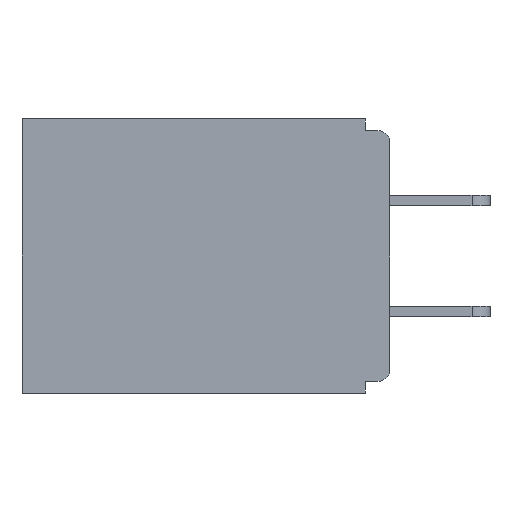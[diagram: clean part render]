
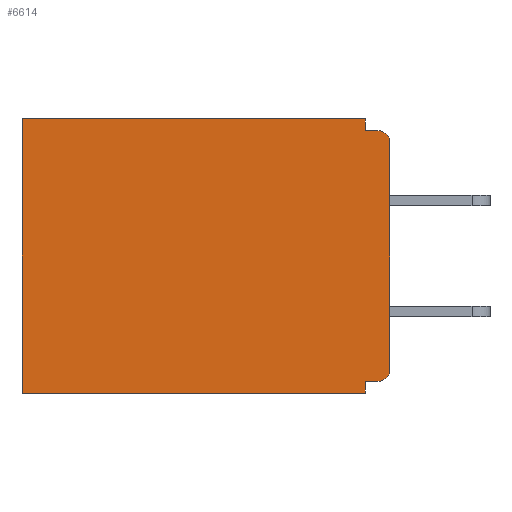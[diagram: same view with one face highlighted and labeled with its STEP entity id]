
A CAD part, left-side view. The second image highlights one B-rep face of the part: STEP entity #6614.
In plain terms, the highlighted planar face has unit normal (-1, 0, 0).
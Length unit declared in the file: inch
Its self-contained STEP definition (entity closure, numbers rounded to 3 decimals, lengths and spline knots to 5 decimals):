
#872 = AXIS2_PLACEMENT_3D ( 'NONE', #21377, #1498, #17815 ) ;
#1228 = DIRECTION ( 'NONE',  ( 0., 1., 0. ) ) ;
#1498 = DIRECTION ( 'NONE',  ( -1., 0., 0. ) ) ;
#2060 = EDGE_LOOP ( 'NONE', ( #9088, #4891, #14933, #8256, #21870, #21727, #25203, #8234, #14014, #2241 ) ) ;
#2160 = VERTEX_POINT ( 'NONE', #13842 ) ;
#2241 = ORIENTED_EDGE ( 'NONE', *, *, #13747, .F. ) ;
#2498 = DIRECTION ( 'NONE',  ( 0., 0., -1. ) ) ;
#3369 = VECTOR ( 'NONE', #23822, 39.37008 ) ;
#3476 = DIRECTION ( 'NONE',  ( 1., 0., 0. ) ) ;
#3759 = VERTEX_POINT ( 'NONE', #11591 ) ;
#3927 = CARTESIAN_POINT ( 'NONE',  ( 0.298, 0., -0.328 ) ) ;
#4252 = EDGE_CURVE ( 'NONE', #3759, #8314, #20548, .T. ) ;
#4494 = LINE ( 'NONE', #11428, #9475 ) ;
#4512 = CARTESIAN_POINT ( 'NONE',  ( 0.298, 0.015, -0.03 ) ) ;
#4557 = EDGE_CURVE ( 'NONE', #3759, #5519, #8683, .T. ) ;
#4628 = LINE ( 'NONE', #11725, #3369 ) ;
#4753 = CARTESIAN_POINT ( 'NONE',  ( 0.298, 0.46, 0. ) ) ;
#4891 = ORIENTED_EDGE ( 'NONE', *, *, #8726, .F. ) ;
#5317 = PLANE ( 'NONE',  #8557 ) ;
#5519 = VERTEX_POINT ( 'NONE', #7289 ) ;
#6614 = ADVANCED_FACE ( 'NONE', ( #15911 ), #5317, .F. ) ;
#7010 = EDGE_CURVE ( 'NONE', #22386, #8711, #13099, .T. ) ;
#7146 = AXIS2_PLACEMENT_3D ( 'NONE', #4512, #18550, #20522 ) ;
#7289 = CARTESIAN_POINT ( 'NONE',  ( 0.298, 0.031, -0.328 ) ) ;
#7302 = DIRECTION ( 'NONE',  ( 0., 0., -1. ) ) ;
#7471 = DIRECTION ( 'NONE',  ( 0., 0., -1. ) ) ;
#7636 = VECTOR ( 'NONE', #1228, 39.37008 ) ;
#8234 = ORIENTED_EDGE ( 'NONE', *, *, #4557, .F. ) ;
#8256 = ORIENTED_EDGE ( 'NONE', *, *, #20867, .T. ) ;
#8286 = LINE ( 'NONE', #14314, #24186 ) ;
#8314 = VERTEX_POINT ( 'NONE', #20433 ) ;
#8557 = AXIS2_PLACEMENT_3D ( 'NONE', #13546, #3476, #7471 ) ;
#8588 = LINE ( 'NONE', #25038, #7636 ) ;
#8683 = LINE ( 'NONE', #3927, #24899 ) ;
#8711 = VERTEX_POINT ( 'NONE', #19725 ) ;
#8726 = EDGE_CURVE ( 'NONE', #21543, #16826, #4628, .T. ) ;
#9088 = ORIENTED_EDGE ( 'NONE', *, *, #20347, .T. ) ;
#9347 = VERTEX_POINT ( 'NONE', #11009 ) ;
#9475 = VECTOR ( 'NONE', #17098, 39.37008 ) ;
#10661 = CARTESIAN_POINT ( 'NONE',  ( 0.298, 0.031, -0.343 ) ) ;
#11009 = CARTESIAN_POINT ( 'NONE',  ( 0.298, 0.46, 0. ) ) ;
#11428 = CARTESIAN_POINT ( 'NONE',  ( 0.298, 0., 0. ) ) ;
#11591 = CARTESIAN_POINT ( 'NONE',  ( 0.298, 0.015, -0.328 ) ) ;
#11686 = EDGE_CURVE ( 'NONE', #9347, #8711, #22696, .T. ) ;
#11725 = CARTESIAN_POINT ( 'NONE',  ( 0.298, 0., -0.015 ) ) ;
#12074 = CARTESIAN_POINT ( 'NONE',  ( 0.298, 0., -0.343 ) ) ;
#13099 = LINE ( 'NONE', #12074, #18102 ) ;
#13546 = CARTESIAN_POINT ( 'NONE',  ( 0.298, 0., 0. ) ) ;
#13747 = EDGE_CURVE ( 'NONE', #2160, #8314, #4494, .T. ) ;
#13807 = DIRECTION ( 'NONE',  ( 0., 1., 0. ) ) ;
#13842 = CARTESIAN_POINT ( 'NONE',  ( 0.298, 0., -0.03 ) ) ;
#14014 = ORIENTED_EDGE ( 'NONE', *, *, #4252, .T. ) ;
#14314 = CARTESIAN_POINT ( 'NONE',  ( 0.298, 0.031, -0.343 ) ) ;
#14933 = ORIENTED_EDGE ( 'NONE', *, *, #20462, .F. ) ;
#15702 = VERTEX_POINT ( 'NONE', #16570 ) ;
#15754 = CIRCLE ( 'NONE', #7146, 0.015 ) ;
#15903 = VECTOR ( 'NONE', #7302, 39.37008 ) ;
#15911 = FACE_OUTER_BOUND ( 'NONE', #2060, .T. ) ;
#16570 = CARTESIAN_POINT ( 'NONE',  ( 0.298, 0.031, 0. ) ) ;
#16826 = VERTEX_POINT ( 'NONE', #17215 ) ;
#17098 = DIRECTION ( 'NONE',  ( 0., 0., -1. ) ) ;
#17215 = CARTESIAN_POINT ( 'NONE',  ( 0.298, 0.015, -0.015 ) ) ;
#17415 = VECTOR ( 'NONE', #24261, 39.37008 ) ;
#17815 = DIRECTION ( 'NONE',  ( 0., 0., -1. ) ) ;
#18102 = VECTOR ( 'NONE', #13807, 39.37008 ) ;
#18550 = DIRECTION ( 'NONE',  ( -1., 0., 0. ) ) ;
#19725 = CARTESIAN_POINT ( 'NONE',  ( 0.298, 0.46, -0.343 ) ) ;
#20212 = CARTESIAN_POINT ( 'NONE',  ( 0.298, 0.031, -0.343 ) ) ;
#20347 = EDGE_CURVE ( 'NONE', #2160, #16826, #15754, .T. ) ;
#20433 = CARTESIAN_POINT ( 'NONE',  ( 0.298, 0., -0.313 ) ) ;
#20462 = EDGE_CURVE ( 'NONE', #15702, #21543, #8286, .T. ) ;
#20522 = DIRECTION ( 'NONE',  ( 0., 0., -1. ) ) ;
#20548 = CIRCLE ( 'NONE', #872, 0.015 ) ;
#20867 = EDGE_CURVE ( 'NONE', #15702, #9347, #8588, .T. ) ;
#21377 = CARTESIAN_POINT ( 'NONE',  ( 0.298, 0.015, -0.313 ) ) ;
#21543 = VERTEX_POINT ( 'NONE', #23667 ) ;
#21727 = ORIENTED_EDGE ( 'NONE', *, *, #7010, .F. ) ;
#21870 = ORIENTED_EDGE ( 'NONE', *, *, #11686, .T. ) ;
#22189 = LINE ( 'NONE', #10661, #15903 ) ;
#22386 = VERTEX_POINT ( 'NONE', #20212 ) ;
#22625 = DIRECTION ( 'NONE',  ( 0., 1., 0. ) ) ;
#22696 = LINE ( 'NONE', #4753, #17415 ) ;
#23020 = EDGE_CURVE ( 'NONE', #5519, #22386, #22189, .T. ) ;
#23667 = CARTESIAN_POINT ( 'NONE',  ( 0.298, 0.031, -0.015 ) ) ;
#23822 = DIRECTION ( 'NONE',  ( 0., -1., 0. ) ) ;
#24186 = VECTOR ( 'NONE', #2498, 39.37008 ) ;
#24261 = DIRECTION ( 'NONE',  ( 0., 0., -1. ) ) ;
#24899 = VECTOR ( 'NONE', #22625, 39.37008 ) ;
#25038 = CARTESIAN_POINT ( 'NONE',  ( 0.298, 0., 0. ) ) ;
#25203 = ORIENTED_EDGE ( 'NONE', *, *, #23020, .F. ) ;
